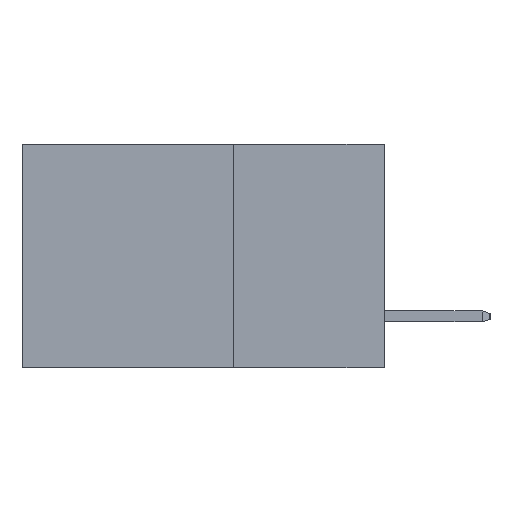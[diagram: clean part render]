
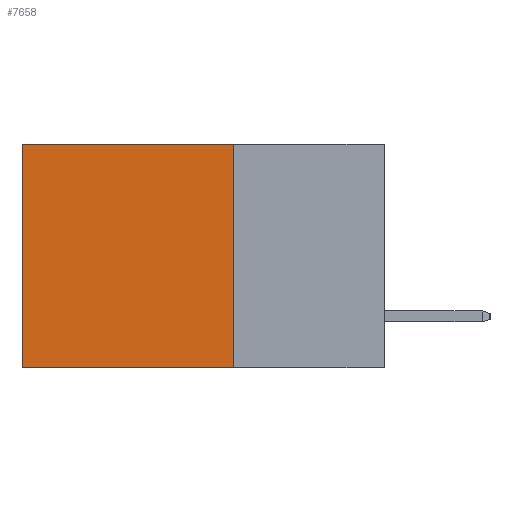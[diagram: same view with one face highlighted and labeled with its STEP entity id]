
A CAD part, left-side view. The second image highlights one B-rep face of the part: STEP entity #7658.
In plain terms, the highlighted planar face has unit normal (-1, 0, 0).
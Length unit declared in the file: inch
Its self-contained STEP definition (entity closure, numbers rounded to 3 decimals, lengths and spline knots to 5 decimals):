
#62 = LINE ( 'NONE', #20189, #22335 ) ;
#311 = CARTESIAN_POINT ( 'NONE',  ( 0.298, 0.6, 0. ) ) ;
#1760 = CARTESIAN_POINT ( 'NONE',  ( 0.298, 0.25, 0. ) ) ;
#2517 = DIRECTION ( 'NONE',  ( 0., 0., -1. ) ) ;
#3230 = ORIENTED_EDGE ( 'NONE', *, *, #22447, .T. ) ;
#4036 = VECTOR ( 'NONE', #2517, 39.37008 ) ;
#4861 = VERTEX_POINT ( 'NONE', #1760 ) ;
#6086 = LINE ( 'NONE', #15102, #27285 ) ;
#7658 = ADVANCED_FACE ( 'NONE', ( #14423 ), #20280, .F. ) ;
#9452 = EDGE_CURVE ( 'NONE', #9586, #26974, #13660, .T. ) ;
#9586 = VERTEX_POINT ( 'NONE', #24595 ) ;
#9815 = CARTESIAN_POINT ( 'NONE',  ( 0.298, 0.6, 0. ) ) ;
#10153 = ORIENTED_EDGE ( 'NONE', *, *, #9452, .F. ) ;
#12312 = VECTOR ( 'NONE', #26841, 39.37008 ) ;
#13628 = VERTEX_POINT ( 'NONE', #9815 ) ;
#13660 = LINE ( 'NONE', #26380, #12312 ) ;
#14423 = FACE_OUTER_BOUND ( 'NONE', #16485, .T. ) ;
#14754 = LINE ( 'NONE', #311, #4036 ) ;
#15102 = CARTESIAN_POINT ( 'NONE',  ( 0.298, 0.25, 0. ) ) ;
#16485 = EDGE_LOOP ( 'NONE', ( #22984, #10153, #25770, #3230 ) ) ;
#18363 = EDGE_CURVE ( 'NONE', #4861, #9586, #6086, .T. ) ;
#18442 = EDGE_CURVE ( 'NONE', #13628, #26974, #14754, .T. ) ;
#19916 = DIRECTION ( 'NONE',  ( 0., 0., -1. ) ) ;
#20015 = DIRECTION ( 'NONE',  ( 1., 0., 0. ) ) ;
#20144 = CARTESIAN_POINT ( 'NONE',  ( 0.298, 0.25, 0. ) ) ;
#20189 = CARTESIAN_POINT ( 'NONE',  ( 0.298, 0.25, 0. ) ) ;
#20280 = PLANE ( 'NONE',  #23024 ) ;
#21627 = DIRECTION ( 'NONE',  ( 0., 0., -1. ) ) ;
#22200 = CARTESIAN_POINT ( 'NONE',  ( 0.298, 0.6, -0.37 ) ) ;
#22335 = VECTOR ( 'NONE', #24455, 39.37008 ) ;
#22447 = EDGE_CURVE ( 'NONE', #4861, #13628, #62, .T. ) ;
#22984 = ORIENTED_EDGE ( 'NONE', *, *, #18442, .T. ) ;
#23024 = AXIS2_PLACEMENT_3D ( 'NONE', #20144, #20015, #19916 ) ;
#24455 = DIRECTION ( 'NONE',  ( 0., 1., 0. ) ) ;
#24595 = CARTESIAN_POINT ( 'NONE',  ( 0.298, 0.25, -0.37 ) ) ;
#25770 = ORIENTED_EDGE ( 'NONE', *, *, #18363, .F. ) ;
#26380 = CARTESIAN_POINT ( 'NONE',  ( 0.298, 0.25, -0.37 ) ) ;
#26841 = DIRECTION ( 'NONE',  ( 0., 1., 0. ) ) ;
#26974 = VERTEX_POINT ( 'NONE', #22200 ) ;
#27285 = VECTOR ( 'NONE', #21627, 39.37008 ) ;
